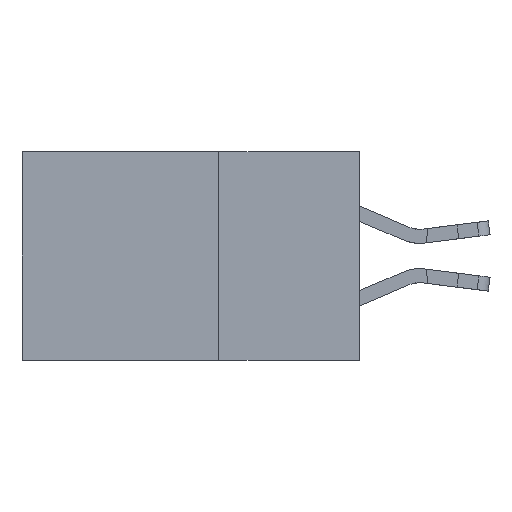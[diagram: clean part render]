
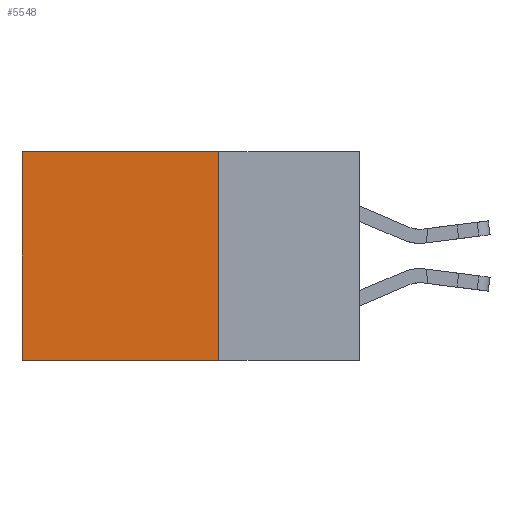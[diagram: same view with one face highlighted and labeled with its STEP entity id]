
A CAD part, left-side view. The second image highlights one B-rep face of the part: STEP entity #5548.
In plain terms, the highlighted planar face has unit normal (-1, 0, 0).
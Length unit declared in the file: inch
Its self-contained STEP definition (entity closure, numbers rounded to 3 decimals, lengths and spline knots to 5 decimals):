
#425 = CARTESIAN_POINT ( 'NONE',  ( 0.2875, 0.25, 0. ) ) ;
#1221 = EDGE_CURVE ( 'NONE', #12982, #22305, #4594, .T. ) ;
#1981 = VERTEX_POINT ( 'NONE', #25881 ) ;
#4594 = LINE ( 'NONE', #22654, #5407 ) ;
#5407 = VECTOR ( 'NONE', #10452, 39.37008 ) ;
#5548 = ADVANCED_FACE ( 'NONE', ( #23694 ), #27086, .F. ) ;
#7446 = CARTESIAN_POINT ( 'NONE',  ( 0.2875, 0.25, 0. ) ) ;
#7777 = ORIENTED_EDGE ( 'NONE', *, *, #9593, .T. ) ;
#8112 = CARTESIAN_POINT ( 'NONE',  ( 0.2875, 0.25, 0. ) ) ;
#9593 = EDGE_CURVE ( 'NONE', #1981, #12982, #23735, .T. ) ;
#9635 = DIRECTION ( 'NONE',  ( 0., 1., 0. ) ) ;
#9854 = AXIS2_PLACEMENT_3D ( 'NONE', #7446, #29478, #15077 ) ;
#9902 = EDGE_CURVE ( 'NONE', #11414, #22305, #28237, .T. ) ;
#10452 = DIRECTION ( 'NONE',  ( 0., 0., -1. ) ) ;
#11414 = VERTEX_POINT ( 'NONE', #17532 ) ;
#11838 = VECTOR ( 'NONE', #18010, 39.37008 ) ;
#11858 = EDGE_CURVE ( 'NONE', #1981, #11414, #30413, .T. ) ;
#12209 = CARTESIAN_POINT ( 'NONE',  ( 0.2875, 0.25, -0.37 ) ) ;
#12982 = VERTEX_POINT ( 'NONE', #24319 ) ;
#15077 = DIRECTION ( 'NONE',  ( 0., 0., -1. ) ) ;
#15951 = ORIENTED_EDGE ( 'NONE', *, *, #11858, .F. ) ;
#17532 = CARTESIAN_POINT ( 'NONE',  ( 0.2875, 0.25, -0.37 ) ) ;
#18010 = DIRECTION ( 'NONE',  ( 0., 0., -1. ) ) ;
#18613 = CARTESIAN_POINT ( 'NONE',  ( 0.2875, 0.6, -0.37 ) ) ;
#22305 = VERTEX_POINT ( 'NONE', #18613 ) ;
#22654 = CARTESIAN_POINT ( 'NONE',  ( 0.2875, 0.6, 0. ) ) ;
#23694 = FACE_OUTER_BOUND ( 'NONE', #27299, .T. ) ;
#23735 = LINE ( 'NONE', #8112, #30137 ) ;
#24319 = CARTESIAN_POINT ( 'NONE',  ( 0.2875, 0.6, 0. ) ) ;
#24730 = ORIENTED_EDGE ( 'NONE', *, *, #9902, .F. ) ;
#25261 = DIRECTION ( 'NONE',  ( 0., 1., 0. ) ) ;
#25881 = CARTESIAN_POINT ( 'NONE',  ( 0.2875, 0.25, 0. ) ) ;
#27086 = PLANE ( 'NONE',  #9854 ) ;
#27299 = EDGE_LOOP ( 'NONE', ( #28530, #24730, #15951, #7777 ) ) ;
#27487 = VECTOR ( 'NONE', #9635, 39.37008 ) ;
#28237 = LINE ( 'NONE', #12209, #27487 ) ;
#28530 = ORIENTED_EDGE ( 'NONE', *, *, #1221, .T. ) ;
#29478 = DIRECTION ( 'NONE',  ( 1., 0., 0. ) ) ;
#30137 = VECTOR ( 'NONE', #25261, 39.37008 ) ;
#30413 = LINE ( 'NONE', #425, #11838 ) ;
